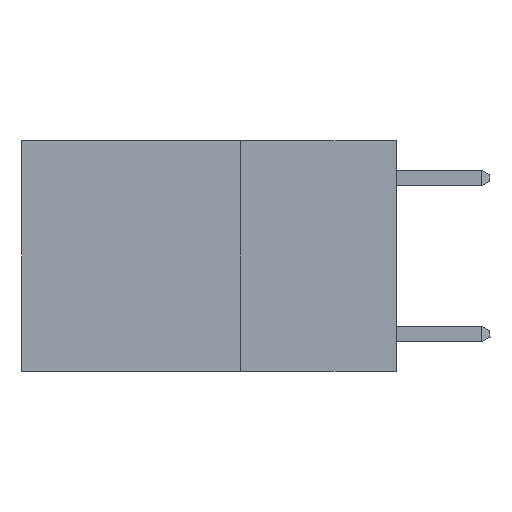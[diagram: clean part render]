
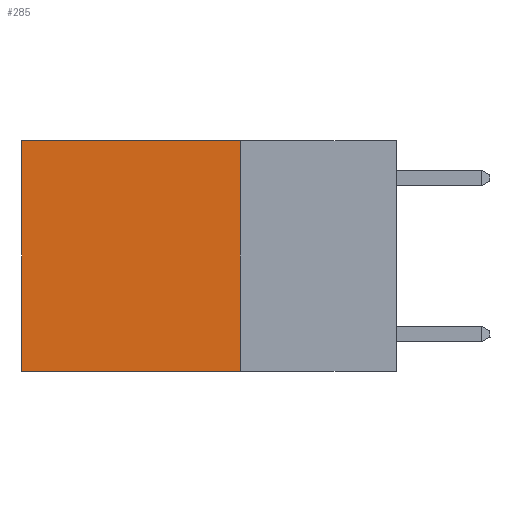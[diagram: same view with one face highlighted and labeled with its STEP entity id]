
A CAD part, left-side view. The second image highlights one B-rep face of the part: STEP entity #285.
In plain terms, the highlighted planar face has unit normal (-1, 0, 0).
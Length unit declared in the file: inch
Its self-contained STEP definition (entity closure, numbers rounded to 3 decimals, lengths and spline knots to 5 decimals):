
#140 = VECTOR ( 'NONE', #19558, 39.37008 ) ;
#285 = ADVANCED_FACE ( 'NONE', ( #14719 ), #5462, .F. ) ;
#618 = CARTESIAN_POINT ( 'NONE',  ( 0.2625, 0.25, -0.37 ) ) ;
#714 = LINE ( 'NONE', #18168, #140 ) ;
#1603 = ORIENTED_EDGE ( 'NONE', *, *, #13528, .F. ) ;
#1794 = AXIS2_PLACEMENT_3D ( 'NONE', #3491, #3317, #6761 ) ;
#2074 = CARTESIAN_POINT ( 'NONE',  ( 0.2625, 0.25, 0. ) ) ;
#2457 = VERTEX_POINT ( 'NONE', #8281 ) ;
#3207 = VECTOR ( 'NONE', #7990, 39.37008 ) ;
#3317 = DIRECTION ( 'NONE',  ( 1., 0., 0. ) ) ;
#3322 = LINE ( 'NONE', #6445, #3207 ) ;
#3491 = CARTESIAN_POINT ( 'NONE',  ( 0.2625, 0.25, 0. ) ) ;
#4602 = VERTEX_POINT ( 'NONE', #18920 ) ;
#4901 = VECTOR ( 'NONE', #17040, 39.37008 ) ;
#5218 = LINE ( 'NONE', #6437, #4901 ) ;
#5254 = ORIENTED_EDGE ( 'NONE', *, *, #7464, .T. ) ;
#5462 = PLANE ( 'NONE',  #1794 ) ;
#5529 = CARTESIAN_POINT ( 'NONE',  ( 0.2625, 0.6, 0. ) ) ;
#6437 = CARTESIAN_POINT ( 'NONE',  ( 0.2625, 0.25, 0. ) ) ;
#6445 = CARTESIAN_POINT ( 'NONE',  ( 0.2625, 0.25, 0. ) ) ;
#6761 = DIRECTION ( 'NONE',  ( 0., 0., -1. ) ) ;
#7464 = EDGE_CURVE ( 'NONE', #14830, #2457, #3322, .T. ) ;
#7990 = DIRECTION ( 'NONE',  ( 0., 1., 0. ) ) ;
#8281 = CARTESIAN_POINT ( 'NONE',  ( 0.2625, 0.6, 0. ) ) ;
#9764 = EDGE_LOOP ( 'NONE', ( #10385, #11846, #1603, #5254 ) ) ;
#10235 = EDGE_CURVE ( 'NONE', #18158, #4602, #714, .T. ) ;
#10319 = VECTOR ( 'NONE', #19114, 39.37008 ) ;
#10385 = ORIENTED_EDGE ( 'NONE', *, *, #17530, .T. ) ;
#10826 = LINE ( 'NONE', #5529, #10319 ) ;
#11846 = ORIENTED_EDGE ( 'NONE', *, *, #10235, .F. ) ;
#13528 = EDGE_CURVE ( 'NONE', #14830, #18158, #5218, .T. ) ;
#14719 = FACE_OUTER_BOUND ( 'NONE', #9764, .T. ) ;
#14830 = VERTEX_POINT ( 'NONE', #2074 ) ;
#17040 = DIRECTION ( 'NONE',  ( 0., 0., -1. ) ) ;
#17530 = EDGE_CURVE ( 'NONE', #2457, #4602, #10826, .T. ) ;
#18158 = VERTEX_POINT ( 'NONE', #618 ) ;
#18168 = CARTESIAN_POINT ( 'NONE',  ( 0.2625, 0.25, -0.37 ) ) ;
#18920 = CARTESIAN_POINT ( 'NONE',  ( 0.2625, 0.6, -0.37 ) ) ;
#19114 = DIRECTION ( 'NONE',  ( 0., 0., -1. ) ) ;
#19558 = DIRECTION ( 'NONE',  ( 0., 1., 0. ) ) ;
